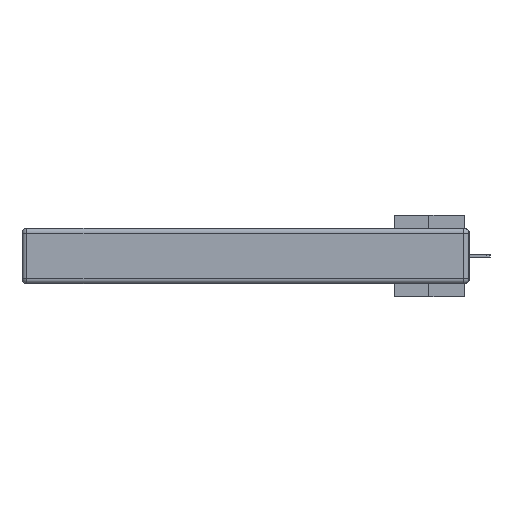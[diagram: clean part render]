
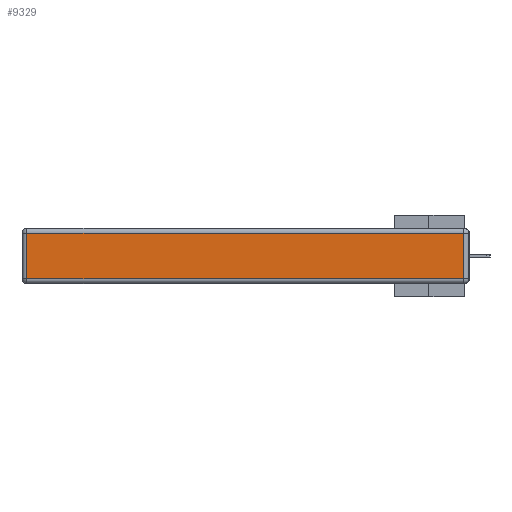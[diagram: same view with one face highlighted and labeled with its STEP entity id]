
A CAD part, left-side view. The second image highlights one B-rep face of the part: STEP entity #9329.
In plain terms, the highlighted planar face has unit normal (-1, 0, 0).
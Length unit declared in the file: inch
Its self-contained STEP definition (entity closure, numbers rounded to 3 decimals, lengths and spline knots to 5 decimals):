
#328 = DIRECTION ( 'NONE',  ( 0., 0., -1. ) ) ;
#1068 = VECTOR ( 'NONE', #18413, 39.37008 ) ;
#2129 = CARTESIAN_POINT ( 'NONE',  ( 0., 2.72, -0.313 ) ) ;
#2392 = VECTOR ( 'NONE', #7198, 39.37008 ) ;
#2551 = EDGE_CURVE ( 'NONE', #25492, #30136, #16268, .T. ) ;
#4415 = FACE_OUTER_BOUND ( 'NONE', #17416, .T. ) ;
#5207 = DIRECTION ( 'NONE',  ( -1., 0., 0. ) ) ;
#5518 = CARTESIAN_POINT ( 'NONE',  ( 0., 0.03, -0.343 ) ) ;
#6042 = EDGE_CURVE ( 'NONE', #33018, #12751, #29533, .T. ) ;
#6481 = EDGE_CURVE ( 'NONE', #12751, #25492, #21891, .T. ) ;
#7198 = DIRECTION ( 'NONE',  ( 0., -1., 0. ) ) ;
#7202 = PLANE ( 'NONE',  #8671 ) ;
#8487 = ORIENTED_EDGE ( 'NONE', *, *, #2551, .T. ) ;
#8671 = AXIS2_PLACEMENT_3D ( 'NONE', #25761, #5207, #20321 ) ;
#9329 = ADVANCED_FACE ( 'NONE', ( #4415 ), #7202, .T. ) ;
#12751 = VERTEX_POINT ( 'NONE', #2129 ) ;
#14134 = ORIENTED_EDGE ( 'NONE', *, *, #17782, .T. ) ;
#16101 = DIRECTION ( 'NONE',  ( 0., 1., 0. ) ) ;
#16268 = LINE ( 'NONE', #5518, #1068 ) ;
#17416 = EDGE_LOOP ( 'NONE', ( #23621, #8487, #14134, #29377 ) ) ;
#17559 = CARTESIAN_POINT ( 'NONE',  ( 0., 0., -0.313 ) ) ;
#17782 = EDGE_CURVE ( 'NONE', #30136, #33018, #22948, .T. ) ;
#18413 = DIRECTION ( 'NONE',  ( 0., 0., 1. ) ) ;
#19553 = VECTOR ( 'NONE', #328, 39.37008 ) ;
#20321 = DIRECTION ( 'NONE',  ( 0., 0., 1. ) ) ;
#21108 = CARTESIAN_POINT ( 'NONE',  ( 0., 2.75, -0.03 ) ) ;
#21891 = LINE ( 'NONE', #17559, #2392 ) ;
#22118 = VECTOR ( 'NONE', #16101, 39.37008 ) ;
#22948 = LINE ( 'NONE', #21108, #22118 ) ;
#23621 = ORIENTED_EDGE ( 'NONE', *, *, #6481, .T. ) ;
#25492 = VERTEX_POINT ( 'NONE', #31582 ) ;
#25761 = CARTESIAN_POINT ( 'NONE',  ( 0., 0., -0.343 ) ) ;
#26287 = CARTESIAN_POINT ( 'NONE',  ( 0., 2.72, -0.343 ) ) ;
#26463 = CARTESIAN_POINT ( 'NONE',  ( 0., 2.72, -0.03 ) ) ;
#27611 = CARTESIAN_POINT ( 'NONE',  ( 0., 0.03, -0.03 ) ) ;
#29377 = ORIENTED_EDGE ( 'NONE', *, *, #6042, .T. ) ;
#29533 = LINE ( 'NONE', #26287, #19553 ) ;
#30136 = VERTEX_POINT ( 'NONE', #27611 ) ;
#31582 = CARTESIAN_POINT ( 'NONE',  ( 0., 0.03, -0.313 ) ) ;
#33018 = VERTEX_POINT ( 'NONE', #26463 ) ;
